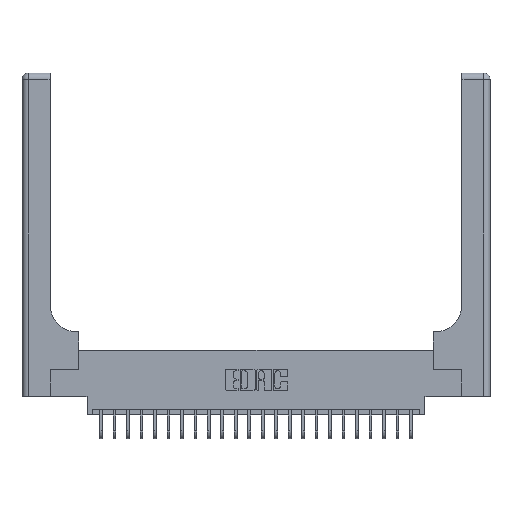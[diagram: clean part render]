
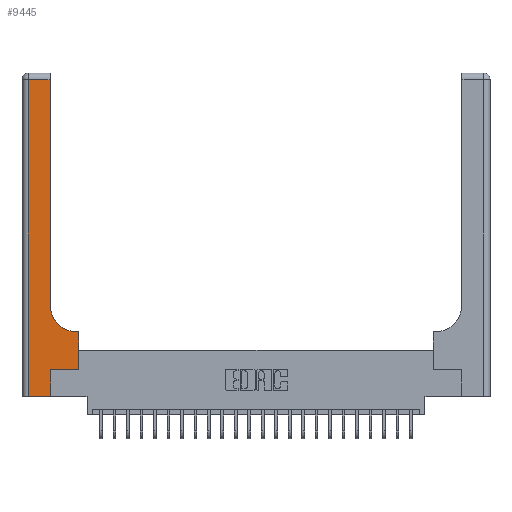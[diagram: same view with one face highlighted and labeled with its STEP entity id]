
A CAD part, top view. The second image highlights one B-rep face of the part: STEP entity #9445.
In plain terms, the highlighted planar face has unit normal (0, 0, 1).
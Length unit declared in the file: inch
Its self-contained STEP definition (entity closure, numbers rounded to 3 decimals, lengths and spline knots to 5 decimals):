
#552 = LINE ( 'NONE', #2387, #12068 ) ;
#570 = LINE ( 'NONE', #8478, #8268 ) ;
#674 = CIRCLE ( 'NONE', #14351, 0.25 ) ;
#947 = DIRECTION ( 'NONE',  ( 0., 1., 0. ) ) ;
#2387 = CARTESIAN_POINT ( 'NONE',  ( 0.265, 0., 0.37 ) ) ;
#2949 = DIRECTION ( 'NONE',  ( 0., 0., -1. ) ) ;
#3436 = DIRECTION ( 'NONE',  ( 0., 1., 0. ) ) ;
#3702 = LINE ( 'NONE', #22677, #24027 ) ;
#3977 = VERTEX_POINT ( 'NONE', #4022 ) ;
#4022 = CARTESIAN_POINT ( 'NONE',  ( 0.265, 0., 0.37 ) ) ;
#4076 = ORIENTED_EDGE ( 'NONE', *, *, #4299, .T. ) ;
#4299 = EDGE_CURVE ( 'NONE', #15984, #21711, #3702, .T. ) ;
#4484 = EDGE_CURVE ( 'NONE', #6989, #14730, #570, .T. ) ;
#4516 = ORIENTED_EDGE ( 'NONE', *, *, #13511, .T. ) ;
#4689 = CARTESIAN_POINT ( 'NONE',  ( 0.51, 0.6, 0.37 ) ) ;
#5402 = CARTESIAN_POINT ( 'NONE',  ( 0., 3., 0.37 ) ) ;
#5739 = CARTESIAN_POINT ( 'NONE',  ( 0.51, 0.85, 0.37 ) ) ;
#6451 = ORIENTED_EDGE ( 'NONE', *, *, #21784, .T. ) ;
#6577 = LINE ( 'NONE', #8654, #20908 ) ;
#6957 = DIRECTION ( 'NONE',  ( -1., 0., 0. ) ) ;
#6989 = VERTEX_POINT ( 'NONE', #9425 ) ;
#7073 = VERTEX_POINT ( 'NONE', #4689 ) ;
#7336 = PLANE ( 'NONE',  #15563 ) ;
#8268 = VECTOR ( 'NONE', #947, 39.37008 ) ;
#8478 = CARTESIAN_POINT ( 'NONE',  ( 0.26, 3., 0.37 ) ) ;
#8654 = CARTESIAN_POINT ( 'NONE',  ( 0.26, 0.6, 0.37 ) ) ;
#8752 = ORIENTED_EDGE ( 'NONE', *, *, #4484, .T. ) ;
#9293 = EDGE_CURVE ( 'NONE', #21711, #7073, #6577, .T. ) ;
#9376 = LINE ( 'NONE', #24804, #15778 ) ;
#9425 = CARTESIAN_POINT ( 'NONE',  ( 0.26, 0.85, 0.37 ) ) ;
#9445 = ADVANCED_FACE ( 'NONE', ( #25124 ), #7336, .F. ) ;
#9696 = LINE ( 'NONE', #23449, #15067 ) ;
#9777 = DIRECTION ( 'NONE',  ( 0., 0., -1. ) ) ;
#9983 = CARTESIAN_POINT ( 'NONE',  ( 0.06, 2.94, 0.37 ) ) ;
#10710 = CARTESIAN_POINT ( 'NONE',  ( 0.26, 2.94, 0.37 ) ) ;
#10779 = ORIENTED_EDGE ( 'NONE', *, *, #9293, .T. ) ;
#12068 = VECTOR ( 'NONE', #14321, 39.37008 ) ;
#13420 = CARTESIAN_POINT ( 'NONE',  ( 0.06, 0., 0.37 ) ) ;
#13468 = VERTEX_POINT ( 'NONE', #9983 ) ;
#13511 = EDGE_CURVE ( 'NONE', #13468, #15983, #19721, .T. ) ;
#13979 = EDGE_CURVE ( 'NONE', #7073, #6989, #674, .T. ) ;
#14120 = VECTOR ( 'NONE', #19423, 39.37008 ) ;
#14321 = DIRECTION ( 'NONE',  ( 0., 1., 0. ) ) ;
#14351 = AXIS2_PLACEMENT_3D ( 'NONE', #5739, #9777, #25593 ) ;
#14730 = VERTEX_POINT ( 'NONE', #10710 ) ;
#15067 = VECTOR ( 'NONE', #19680, 39.37008 ) ;
#15356 = DIRECTION ( 'NONE',  ( 1., 0., 0. ) ) ;
#15563 = AXIS2_PLACEMENT_3D ( 'NONE', #5402, #2949, #6957 ) ;
#15778 = VECTOR ( 'NONE', #15356, 39.37008 ) ;
#15974 = ORIENTED_EDGE ( 'NONE', *, *, #21108, .T. ) ;
#15983 = VERTEX_POINT ( 'NONE', #13420 ) ;
#15984 = VERTEX_POINT ( 'NONE', #16934 ) ;
#16934 = CARTESIAN_POINT ( 'NONE',  ( 0.528, 0.25, 0.37 ) ) ;
#17608 = LINE ( 'NONE', #19299, #14120 ) ;
#18739 = CARTESIAN_POINT ( 'NONE',  ( 0.265, 0.25, 0.37 ) ) ;
#19299 = CARTESIAN_POINT ( 'NONE',  ( 0., 2.94, 0.37 ) ) ;
#19340 = CARTESIAN_POINT ( 'NONE',  ( 0.06, 3., 0.37 ) ) ;
#19423 = DIRECTION ( 'NONE',  ( -1., 0., 0. ) ) ;
#19466 = ORIENTED_EDGE ( 'NONE', *, *, #24227, .T. ) ;
#19680 = DIRECTION ( 'NONE',  ( 1., 0., 0. ) ) ;
#19721 = LINE ( 'NONE', #19340, #24962 ) ;
#20179 = VERTEX_POINT ( 'NONE', #18739 ) ;
#20699 = EDGE_CURVE ( 'NONE', #15983, #3977, #9376, .T. ) ;
#20908 = VECTOR ( 'NONE', #24488, 39.37008 ) ;
#21108 = EDGE_CURVE ( 'NONE', #14730, #13468, #17608, .T. ) ;
#21711 = VERTEX_POINT ( 'NONE', #21952 ) ;
#21784 = EDGE_CURVE ( 'NONE', #3977, #20179, #552, .T. ) ;
#21952 = CARTESIAN_POINT ( 'NONE',  ( 0.528, 0.6, 0.37 ) ) ;
#22677 = CARTESIAN_POINT ( 'NONE',  ( 0.528, 0.25, 0.37 ) ) ;
#22864 = ORIENTED_EDGE ( 'NONE', *, *, #13979, .T. ) ;
#23223 = DIRECTION ( 'NONE',  ( 0., -1., 0. ) ) ;
#23357 = EDGE_LOOP ( 'NONE', ( #8752, #15974, #4516, #23619, #6451, #19466, #4076, #10779, #22864 ) ) ;
#23449 = CARTESIAN_POINT ( 'NONE',  ( 0.265, 0.25, 0.37 ) ) ;
#23619 = ORIENTED_EDGE ( 'NONE', *, *, #20699, .T. ) ;
#24027 = VECTOR ( 'NONE', #3436, 39.37008 ) ;
#24227 = EDGE_CURVE ( 'NONE', #20179, #15984, #9696, .T. ) ;
#24488 = DIRECTION ( 'NONE',  ( -1., 0., 0. ) ) ;
#24804 = CARTESIAN_POINT ( 'NONE',  ( 0., 0., 0.37 ) ) ;
#24962 = VECTOR ( 'NONE', #23223, 39.37008 ) ;
#25124 = FACE_OUTER_BOUND ( 'NONE', #23357, .T. ) ;
#25593 = DIRECTION ( 'NONE',  ( 1., 0., 0. ) ) ;
